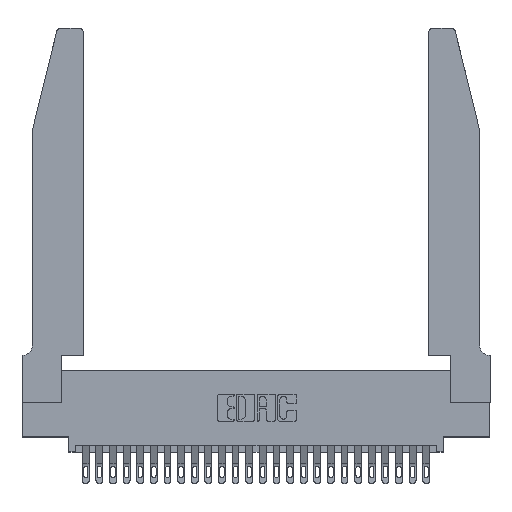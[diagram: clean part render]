
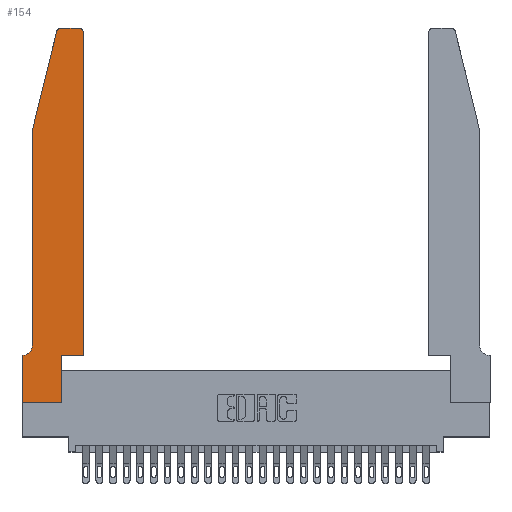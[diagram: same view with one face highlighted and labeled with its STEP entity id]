
A CAD part, top view. The second image highlights one B-rep face of the part: STEP entity #154.
In plain terms, the highlighted planar face has unit normal (0, 0, 1).
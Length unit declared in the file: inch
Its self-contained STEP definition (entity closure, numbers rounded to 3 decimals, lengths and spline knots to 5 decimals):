
#154 = ADVANCED_FACE ( 'NONE', ( #18685 ), #10749, .T. ) ;
#155 = DIRECTION ( 'NONE',  ( 0., 0., 1. ) ) ;
#323 = CARTESIAN_POINT ( 'NONE',  ( 0.0755, 2., 0.37 ) ) ;
#415 = CARTESIAN_POINT ( 'NONE',  ( 0.284, 2.75, 0.37 ) ) ;
#554 = DIRECTION ( 'NONE',  ( -1., 0., 0. ) ) ;
#1195 = CARTESIAN_POINT ( 'NONE',  ( 0.4505, 0.35, 0.37 ) ) ;
#1314 = DIRECTION ( 'NONE',  ( 0., 1., 0. ) ) ;
#1426 = LINE ( 'NONE', #17788, #5840 ) ;
#1427 = EDGE_CURVE ( 'NONE', #8446, #1854, #3099, .T. ) ;
#1463 = EDGE_CURVE ( 'NONE', #1854, #2703, #12540, .T. ) ;
#1515 = DIRECTION ( 'NONE',  ( 0., -1., 0. ) ) ;
#1538 = CARTESIAN_POINT ( 'NONE',  ( 0.4205, 2.75, 0.37 ) ) ;
#1854 = VERTEX_POINT ( 'NONE', #18729 ) ;
#2243 = CARTESIAN_POINT ( 'NONE',  ( 0.0755, 0.42, 0.37 ) ) ;
#2247 = EDGE_CURVE ( 'NONE', #13526, #25717, #4406, .T. ) ;
#2520 = EDGE_CURVE ( 'NONE', #19931, #8446, #9747, .T. ) ;
#2563 = DIRECTION ( 'NONE',  ( 0., 0., -1. ) ) ;
#2701 = CARTESIAN_POINT ( 'NONE',  ( 0.0755, 2., 0.37 ) ) ;
#2703 = VERTEX_POINT ( 'NONE', #1538 ) ;
#3099 = LINE ( 'NONE', #20447, #13244 ) ;
#3233 = VECTOR ( 'NONE', #19763, 39.37008 ) ;
#3306 = ORIENTED_EDGE ( 'NONE', *, *, #1463, .T. ) ;
#4109 = CARTESIAN_POINT ( 'NONE',  ( 0.4205, 2.72, 0.37 ) ) ;
#4393 = DIRECTION ( 'NONE',  ( 0., 0., 1. ) ) ;
#4406 = LINE ( 'NONE', #5382, #20865 ) ;
#5240 = CARTESIAN_POINT ( 'NONE',  ( 0.0055, 0.35, 0.37 ) ) ;
#5382 = CARTESIAN_POINT ( 'NONE',  ( 0., 0., 0.37 ) ) ;
#5840 = VECTOR ( 'NONE', #554, 39.37008 ) ;
#6142 = EDGE_CURVE ( 'NONE', #25717, #17608, #22047, .T. ) ;
#6438 = EDGE_CURVE ( 'NONE', #13733, #24432, #16069, .T. ) ;
#7065 = DIRECTION ( 'NONE',  ( 1., 0., 0. ) ) ;
#7326 = ORIENTED_EDGE ( 'NONE', *, *, #8164, .T. ) ;
#7614 = AXIS2_PLACEMENT_3D ( 'NONE', #4109, #4393, #7065 ) ;
#7639 = CARTESIAN_POINT ( 'NONE',  ( 0.2865, 0., 0.37 ) ) ;
#8164 = EDGE_CURVE ( 'NONE', #25542, #14945, #18652, .T. ) ;
#8446 = VERTEX_POINT ( 'NONE', #1195 ) ;
#9747 = LINE ( 'NONE', #22324, #21178 ) ;
#9825 = VECTOR ( 'NONE', #21938, 39.37008 ) ;
#10749 = PLANE ( 'NONE',  #25513 ) ;
#11324 = VECTOR ( 'NONE', #12467, 39.37008 ) ;
#11712 = ORIENTED_EDGE ( 'NONE', *, *, #26370, .T. ) ;
#11777 = VECTOR ( 'NONE', #15034, 39.37008 ) ;
#12453 = LINE ( 'NONE', #12852, #11777 ) ;
#12467 = DIRECTION ( 'NONE',  ( 1., 0., 0. ) ) ;
#12540 = CIRCLE ( 'NONE', #7614, 0.03 ) ;
#12745 = ORIENTED_EDGE ( 'NONE', *, *, #2520, .T. ) ;
#12852 = CARTESIAN_POINT ( 'NONE',  ( 0.2605, 2.75, 0.37 ) ) ;
#13165 = CARTESIAN_POINT ( 'NONE',  ( 0.284, 2.72, 0.37 ) ) ;
#13244 = VECTOR ( 'NONE', #24685, 39.37008 ) ;
#13497 = EDGE_CURVE ( 'NONE', #17608, #19931, #15188, .T. ) ;
#13526 = VERTEX_POINT ( 'NONE', #18597 ) ;
#13733 = VERTEX_POINT ( 'NONE', #19218 ) ;
#13754 = CARTESIAN_POINT ( 'NONE',  ( 0.2865, 0.35, 0.37 ) ) ;
#13821 = AXIS2_PLACEMENT_3D ( 'NONE', #13165, #155, #15328 ) ;
#14451 = ORIENTED_EDGE ( 'NONE', *, *, #22497, .T. ) ;
#14945 = VERTEX_POINT ( 'NONE', #5240 ) ;
#15034 = DIRECTION ( 'NONE',  ( -1., 0., 0. ) ) ;
#15188 = LINE ( 'NONE', #26984, #19524 ) ;
#15328 = DIRECTION ( 'NONE',  ( 1., 0., 0. ) ) ;
#15439 = ORIENTED_EDGE ( 'NONE', *, *, #18935, .T. ) ;
#15492 = CARTESIAN_POINT ( 'NONE',  ( 0.0055, 0.42, 0.37 ) ) ;
#15636 = DIRECTION ( 'NONE',  ( 1., 0., 0. ) ) ;
#16069 = LINE ( 'NONE', #323, #3233 ) ;
#17139 = ORIENTED_EDGE ( 'NONE', *, *, #13497, .T. ) ;
#17608 = VERTEX_POINT ( 'NONE', #7639 ) ;
#17665 = DIRECTION ( 'NONE',  ( -1., 0., 0. ) ) ;
#17788 = CARTESIAN_POINT ( 'NONE',  ( 0.0755, 0.35, 0.37 ) ) ;
#18016 = CARTESIAN_POINT ( 'NONE',  ( 0., 0.35, 0.37 ) ) ;
#18056 = DIRECTION ( 'NONE',  ( 0., 0., 1. ) ) ;
#18597 = CARTESIAN_POINT ( 'NONE',  ( 0., 0.35, 0.37 ) ) ;
#18652 = CIRCLE ( 'NONE', #23326, 0.07 ) ;
#18685 = FACE_OUTER_BOUND ( 'NONE', #23978, .T. ) ;
#18729 = CARTESIAN_POINT ( 'NONE',  ( 0.4505, 2.72, 0.37 ) ) ;
#18935 = EDGE_CURVE ( 'NONE', #2703, #24004, #12453, .T. ) ;
#19218 = CARTESIAN_POINT ( 'NONE',  ( 0.25487, 2.72718, 0.37 ) ) ;
#19524 = VECTOR ( 'NONE', #1314, 39.37008 ) ;
#19733 = CARTESIAN_POINT ( 'NONE',  ( 0.0755, 2., 0.37 ) ) ;
#19763 = DIRECTION ( 'NONE',  ( -0.239, -0.971, 0. ) ) ;
#19931 = VERTEX_POINT ( 'NONE', #13754 ) ;
#20447 = CARTESIAN_POINT ( 'NONE',  ( 0.4505, 0.35, 0.37 ) ) ;
#20525 = CIRCLE ( 'NONE', #13821, 0.03 ) ;
#20865 = VECTOR ( 'NONE', #1515, 39.37008 ) ;
#21178 = VECTOR ( 'NONE', #23986, 39.37008 ) ;
#21257 = LINE ( 'NONE', #2701, #9825 ) ;
#21436 = ORIENTED_EDGE ( 'NONE', *, *, #6142, .T. ) ;
#21744 = ORIENTED_EDGE ( 'NONE', *, *, #25005, .T. ) ;
#21938 = DIRECTION ( 'NONE',  ( 0., -1., 0. ) ) ;
#22047 = LINE ( 'NONE', #23100, #11324 ) ;
#22156 = CARTESIAN_POINT ( 'NONE',  ( 0., 0., 0.37 ) ) ;
#22324 = CARTESIAN_POINT ( 'NONE',  ( 0.4505, 0.35, 0.37 ) ) ;
#22497 = EDGE_CURVE ( 'NONE', #14945, #13526, #1426, .T. ) ;
#23100 = CARTESIAN_POINT ( 'NONE',  ( 0., 0., 0.37 ) ) ;
#23326 = AXIS2_PLACEMENT_3D ( 'NONE', #15492, #2563, #17665 ) ;
#23978 = EDGE_LOOP ( 'NONE', ( #15439, #21744, #27367, #11712, #7326, #14451, #26388, #21436, #17139, #12745, #24753, #3306 ) ) ;
#23986 = DIRECTION ( 'NONE',  ( 1., 0., 0. ) ) ;
#24004 = VERTEX_POINT ( 'NONE', #415 ) ;
#24432 = VERTEX_POINT ( 'NONE', #19733 ) ;
#24685 = DIRECTION ( 'NONE',  ( 0., 1., 0. ) ) ;
#24753 = ORIENTED_EDGE ( 'NONE', *, *, #1427, .T. ) ;
#25005 = EDGE_CURVE ( 'NONE', #24004, #13733, #20525, .T. ) ;
#25513 = AXIS2_PLACEMENT_3D ( 'NONE', #18016, #18056, #15636 ) ;
#25542 = VERTEX_POINT ( 'NONE', #2243 ) ;
#25717 = VERTEX_POINT ( 'NONE', #22156 ) ;
#26370 = EDGE_CURVE ( 'NONE', #24432, #25542, #21257, .T. ) ;
#26388 = ORIENTED_EDGE ( 'NONE', *, *, #2247, .T. ) ;
#26984 = CARTESIAN_POINT ( 'NONE',  ( 0.2865, 0.35, 0.37 ) ) ;
#27367 = ORIENTED_EDGE ( 'NONE', *, *, #6438, .T. ) ;
